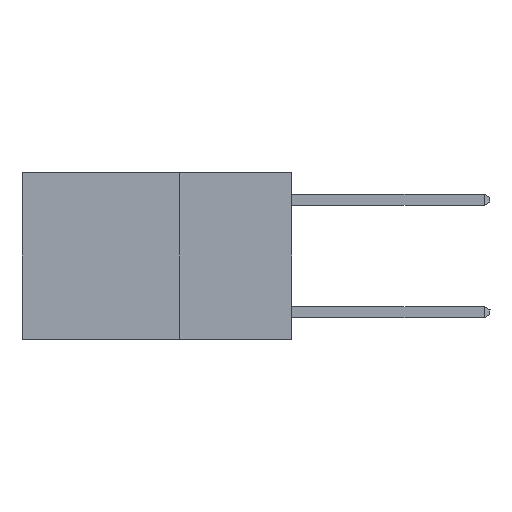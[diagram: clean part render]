
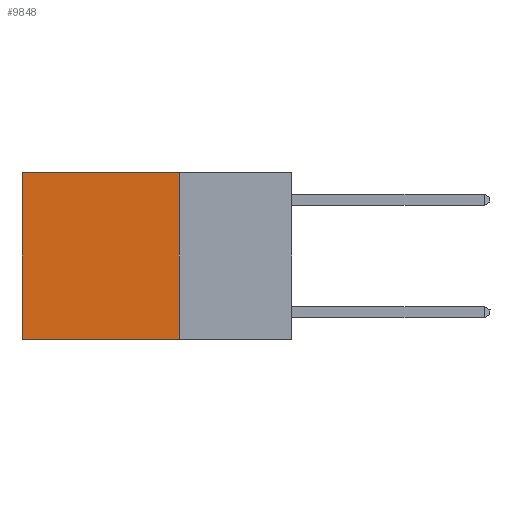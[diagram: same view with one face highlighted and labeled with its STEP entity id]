
A CAD part, left-side view. The second image highlights one B-rep face of the part: STEP entity #9848.
In plain terms, the highlighted planar face has unit normal (-1, 0, 0).
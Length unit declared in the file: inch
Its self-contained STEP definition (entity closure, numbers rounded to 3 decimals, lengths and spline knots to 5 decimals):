
#1173 = CARTESIAN_POINT ( 'NONE',  ( 0.2625, 0.6, -0.37 ) ) ;
#1387 = VECTOR ( 'NONE', #4834, 39.37008 ) ;
#1426 = ORIENTED_EDGE ( 'NONE', *, *, #10445, .F. ) ;
#1504 = CARTESIAN_POINT ( 'NONE',  ( 0.2625, 0.6, 0. ) ) ;
#2258 = DIRECTION ( 'NONE',  ( 0., 1., 0. ) ) ;
#2982 = VECTOR ( 'NONE', #5955, 39.37008 ) ;
#3452 = ORIENTED_EDGE ( 'NONE', *, *, #13422, .T. ) ;
#3799 = LINE ( 'NONE', #23206, #2982 ) ;
#3921 = EDGE_LOOP ( 'NONE', ( #24371, #1426, #19480, #3452 ) ) ;
#4834 = DIRECTION ( 'NONE',  ( 0., 1., 0. ) ) ;
#5441 = VERTEX_POINT ( 'NONE', #1173 ) ;
#5955 = DIRECTION ( 'NONE',  ( 0., 0., -1. ) ) ;
#7211 = DIRECTION ( 'NONE',  ( 1., 0., 0. ) ) ;
#9848 = ADVANCED_FACE ( 'NONE', ( #18699 ), #14532, .F. ) ;
#10309 = CARTESIAN_POINT ( 'NONE',  ( 0.2625, 0.25, -0.37 ) ) ;
#10445 = EDGE_CURVE ( 'NONE', #28025, #5441, #21324, .T. ) ;
#10804 = CARTESIAN_POINT ( 'NONE',  ( 0.2625, 0.25, 0. ) ) ;
#11059 = VECTOR ( 'NONE', #2258, 39.37008 ) ;
#11464 = VERTEX_POINT ( 'NONE', #10804 ) ;
#12539 = VERTEX_POINT ( 'NONE', #1504 ) ;
#13422 = EDGE_CURVE ( 'NONE', #11464, #12539, #17565, .T. ) ;
#14532 = PLANE ( 'NONE',  #20409 ) ;
#14609 = VECTOR ( 'NONE', #31678, 39.37008 ) ;
#17095 = CARTESIAN_POINT ( 'NONE',  ( 0.2625, 0.25, 0. ) ) ;
#17279 = CARTESIAN_POINT ( 'NONE',  ( 0.2625, 0.25, -0.37 ) ) ;
#17565 = LINE ( 'NONE', #31510, #11059 ) ;
#18336 = EDGE_CURVE ( 'NONE', #12539, #5441, #21090, .T. ) ;
#18699 = FACE_OUTER_BOUND ( 'NONE', #3921, .T. ) ;
#19480 = ORIENTED_EDGE ( 'NONE', *, *, #20656, .F. ) ;
#20409 = AXIS2_PLACEMENT_3D ( 'NONE', #17095, #7211, #24381 ) ;
#20656 = EDGE_CURVE ( 'NONE', #11464, #28025, #3799, .T. ) ;
#21090 = LINE ( 'NONE', #29370, #14609 ) ;
#21324 = LINE ( 'NONE', #17279, #1387 ) ;
#23206 = CARTESIAN_POINT ( 'NONE',  ( 0.2625, 0.25, 0. ) ) ;
#24371 = ORIENTED_EDGE ( 'NONE', *, *, #18336, .T. ) ;
#24381 = DIRECTION ( 'NONE',  ( 0., 0., -1. ) ) ;
#28025 = VERTEX_POINT ( 'NONE', #10309 ) ;
#29370 = CARTESIAN_POINT ( 'NONE',  ( 0.2625, 0.6, 0. ) ) ;
#31510 = CARTESIAN_POINT ( 'NONE',  ( 0.2625, 0.25, 0. ) ) ;
#31678 = DIRECTION ( 'NONE',  ( 0., 0., -1. ) ) ;
